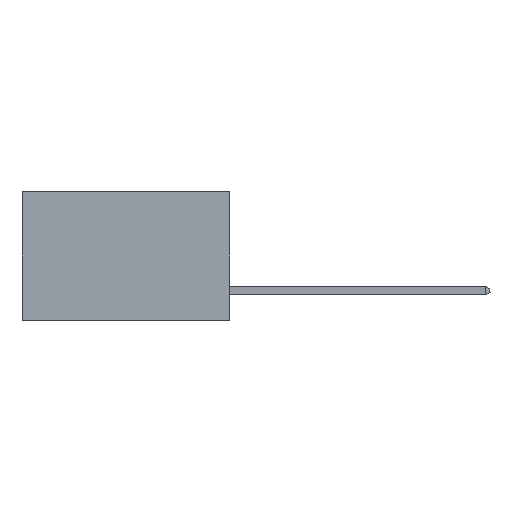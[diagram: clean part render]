
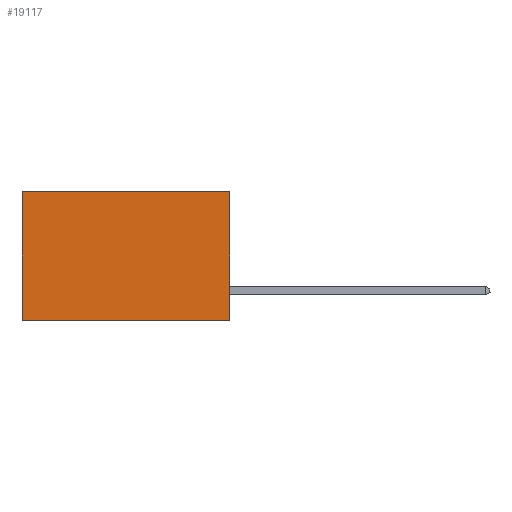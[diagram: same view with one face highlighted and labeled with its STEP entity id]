
A CAD part, left-side view. The second image highlights one B-rep face of the part: STEP entity #19117.
In plain terms, the highlighted planar face has unit normal (-1, 0, 0).
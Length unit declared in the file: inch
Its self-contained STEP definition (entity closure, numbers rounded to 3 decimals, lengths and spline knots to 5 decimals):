
#409 = ORIENTED_EDGE ( 'NONE', *, *, #14073, .T. ) ;
#418 = DIRECTION ( 'NONE',  ( 1., 0., 0. ) ) ;
#2009 = DIRECTION ( 'NONE',  ( 0., 0., -1. ) ) ;
#2499 = AXIS2_PLACEMENT_3D ( 'NONE', #23477, #418, #8616 ) ;
#3132 = ORIENTED_EDGE ( 'NONE', *, *, #11654, .T. ) ;
#3556 = LINE ( 'NONE', #6341, #4515 ) ;
#4515 = VECTOR ( 'NONE', #25525, 39.37008 ) ;
#4716 = PLANE ( 'NONE',  #2499 ) ;
#4731 = CARTESIAN_POINT ( 'NONE',  ( 0.298, 0., -0.37 ) ) ;
#5682 = LINE ( 'NONE', #26594, #12627 ) ;
#6341 = CARTESIAN_POINT ( 'NONE',  ( 0.298, 0., 0. ) ) ;
#6406 = EDGE_CURVE ( 'NONE', #22575, #6975, #3556, .T. ) ;
#6975 = VERTEX_POINT ( 'NONE', #4731 ) ;
#7175 = CARTESIAN_POINT ( 'NONE',  ( 0.298, 0.6, 0. ) ) ;
#8616 = DIRECTION ( 'NONE',  ( 0., 0., -1. ) ) ;
#9547 = VECTOR ( 'NONE', #2009, 39.37008 ) ;
#9761 = DIRECTION ( 'NONE',  ( 0., 1., 0. ) ) ;
#9904 = LINE ( 'NONE', #23111, #25991 ) ;
#10936 = FACE_OUTER_BOUND ( 'NONE', #21607, .T. ) ;
#11654 = EDGE_CURVE ( 'NONE', #22575, #24151, #5682, .T. ) ;
#12413 = CARTESIAN_POINT ( 'NONE',  ( 0.298, 0., 0. ) ) ;
#12525 = CARTESIAN_POINT ( 'NONE',  ( 0.298, 0.6, 0. ) ) ;
#12627 = VECTOR ( 'NONE', #9761, 39.37008 ) ;
#14073 = EDGE_CURVE ( 'NONE', #24151, #23393, #26326, .T. ) ;
#14690 = DIRECTION ( 'NONE',  ( 0., 1., 0. ) ) ;
#15860 = CARTESIAN_POINT ( 'NONE',  ( 0.298, 0.6, -0.37 ) ) ;
#17713 = ORIENTED_EDGE ( 'NONE', *, *, #6406, .F. ) ;
#19117 = ADVANCED_FACE ( 'NONE', ( #10936 ), #4716, .F. ) ;
#21607 = EDGE_LOOP ( 'NONE', ( #409, #26249, #17713, #3132 ) ) ;
#22204 = EDGE_CURVE ( 'NONE', #6975, #23393, #9904, .T. ) ;
#22575 = VERTEX_POINT ( 'NONE', #12413 ) ;
#23111 = CARTESIAN_POINT ( 'NONE',  ( 0.298, 0., -0.37 ) ) ;
#23393 = VERTEX_POINT ( 'NONE', #15860 ) ;
#23477 = CARTESIAN_POINT ( 'NONE',  ( 0.298, 0., 0. ) ) ;
#24151 = VERTEX_POINT ( 'NONE', #7175 ) ;
#25525 = DIRECTION ( 'NONE',  ( 0., 0., -1. ) ) ;
#25991 = VECTOR ( 'NONE', #14690, 39.37008 ) ;
#26249 = ORIENTED_EDGE ( 'NONE', *, *, #22204, .F. ) ;
#26326 = LINE ( 'NONE', #12525, #9547 ) ;
#26594 = CARTESIAN_POINT ( 'NONE',  ( 0.298, 0., 0. ) ) ;
